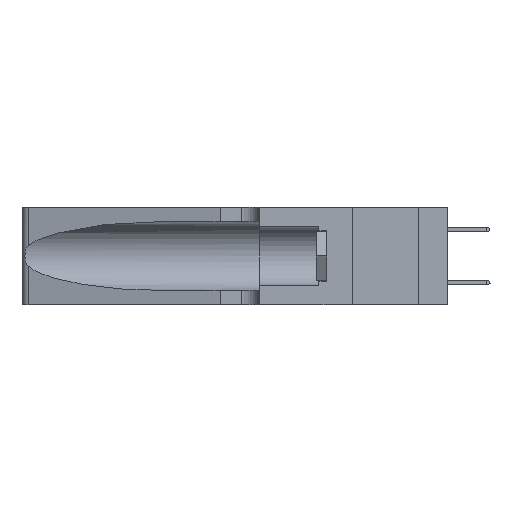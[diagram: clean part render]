
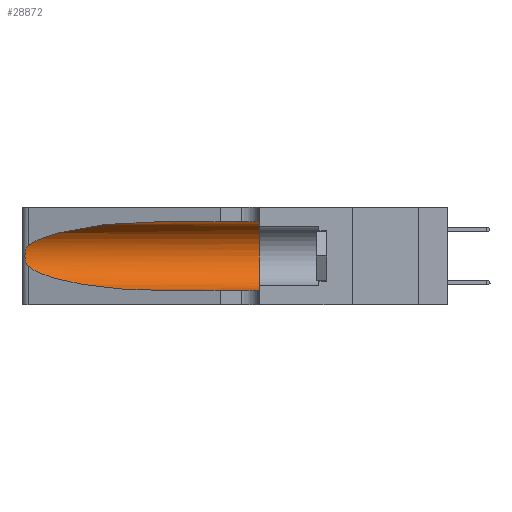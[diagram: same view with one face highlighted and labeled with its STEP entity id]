
A CAD part, left-side view. The second image highlights one B-rep face of the part: STEP entity #28872.
In plain terms, the highlighted cylindrical face has radius 3.308 mm (diameter 6.617 mm), a partial arc.
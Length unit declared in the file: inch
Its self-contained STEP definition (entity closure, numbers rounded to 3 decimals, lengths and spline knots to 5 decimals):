
#1121 = EDGE_CURVE ( 'NONE', #14903, #35474, #17194, .T. ) ;
#1436 = DIRECTION ( 'NONE',  ( 0., -1., 0. ) ) ;
#2239 =( BOUNDED_CURVE ( )  B_SPLINE_CURVE ( 3, ( #35504, #18573, #24895, #11914 ),
 .UNSPECIFIED., .F., .F. ) 
 B_SPLINE_CURVE_WITH_KNOTS ( ( 4, 4 ),
 ( 1.5708, 2.84003 ),
 .UNSPECIFIED. ) 
 CURVE ( )  GEOMETRIC_REPRESENTATION_ITEM ( )  RATIONAL_B_SPLINE_CURVE ( ( 1., 0.87, 0.87, 1. ) ) 
 REPRESENTATION_ITEM ( '' )  );
#2908 = CARTESIAN_POINT ( 'NONE',  ( 0.25487, 1.22718, 0.14631 ) ) ;
#4301 = CARTESIAN_POINT ( 'NONE',  ( 0.25789, 1.23486, 0.15765 ) ) ;
#4594 = CARTESIAN_POINT ( 'NONE',  ( 0.26075, 1.23896, 0.178 ) ) ;
#4607 = CARTESIAN_POINT ( 'NONE',  ( 0.1305, 0.72297, 0.05475 ) ) ;
#5167 = VERTEX_POINT ( 'NONE', #35663 ) ;
#6373 = EDGE_CURVE ( 'NONE', #39963, #35474, #22279, .T. ) ;
#7289 = EDGE_CURVE ( 'NONE', #42876, #39963, #41157, .T. ) ;
#7400 = EDGE_CURVE ( 'NONE', #5167, #22324, #35606, .T. ) ;
#7679 = CARTESIAN_POINT ( 'NONE',  ( 0.25555, 1.22993, 0.14849 ) ) ;
#8824 = ORIENTED_EDGE ( 'NONE', *, *, #1121, .T. ) ;
#9812 = AXIS2_PLACEMENT_3D ( 'NONE', #29751, #33416, #30193 ) ;
#10909 = CARTESIAN_POINT ( 'NONE',  ( 0.26017, 1.23833, 0.17102 ) ) ;
#11914 = CARTESIAN_POINT ( 'NONE',  ( 0.25487, 1.22718, 0.22369 ) ) ;
#13671 = EDGE_LOOP ( 'NONE', ( #27411, #39486, #29930, #8824, #27337, #23279 ) ) ;
#14017 = CARTESIAN_POINT ( 'NONE',  ( 0.25787, 1.23484, 0.2124 ) ) ;
#14903 = VERTEX_POINT ( 'NONE', #4607 ) ;
#15206 =( BOUNDED_CURVE ( )  B_SPLINE_CURVE ( 3, ( #22423, #25263, #18950, #25704 ),
 .UNSPECIFIED., .F., .F. ) 
 B_SPLINE_CURVE_WITH_KNOTS ( ( 4, 4 ),
 ( 3.44316, 4.71239 ),
 .UNSPECIFIED. ) 
 CURVE ( )  GEOMETRIC_REPRESENTATION_ITEM ( )  RATIONAL_B_SPLINE_CURVE ( ( 1., 0.87, 0.87, 1. ) ) 
 REPRESENTATION_ITEM ( '' )  );
#15389 = AXIS2_PLACEMENT_3D ( 'NONE', #18249, #1436, #25156 ) ;
#15490 = CARTESIAN_POINT ( 'NONE',  ( 0.1305, 1.61858, 0.05475 ) ) ;
#17113 = CARTESIAN_POINT ( 'NONE',  ( 0.25639, 1.23184, 0.21858 ) ) ;
#17194 = LINE ( 'NONE', #15490, #34217 ) ;
#17401 = CARTESIAN_POINT ( 'NONE',  ( 0.25854, 1.2359, 0.20912 ) ) ;
#17864 = VECTOR ( 'NONE', #36805, 39.37008 ) ;
#18249 = CARTESIAN_POINT ( 'NONE',  ( 0.1305, 1.61858, 0.185 ) ) ;
#18559 = CYLINDRICAL_SURFACE ( 'NONE', #15389, 0.13025 ) ;
#18573 = CARTESIAN_POINT ( 'NONE',  ( 0.18966, 0.96281, 0.31525 ) ) ;
#18950 = CARTESIAN_POINT ( 'NONE',  ( 0.18966, 0.96281, 0.05475 ) ) ;
#20403 = CARTESIAN_POINT ( 'NONE',  ( 0.1305, 0.35, 0.31525 ) ) ;
#20869 = CARTESIAN_POINT ( 'NONE',  ( 0.25555, 1.22994, 0.2215 ) ) ;
#22206 = EDGE_CURVE ( 'NONE', #42876, #5167, #2239, .T. ) ;
#22279 = CIRCLE ( 'NONE', #9812, 0.13025 ) ;
#22324 = VERTEX_POINT ( 'NONE', #2908 ) ;
#22423 = CARTESIAN_POINT ( 'NONE',  ( 0.25487, 1.22718, 0.14631 ) ) ;
#23279 = ORIENTED_EDGE ( 'NONE', *, *, #7289, .F. ) ;
#24479 = CARTESIAN_POINT ( 'NONE',  ( 0.26018, 1.23835, 0.19895 ) ) ;
#24771 = CARTESIAN_POINT ( 'NONE',  ( 0.25639, 1.23186, 0.15144 ) ) ;
#24895 = CARTESIAN_POINT ( 'NONE',  ( 0.2373, 1.15595, 0.28018 ) ) ;
#25156 = DIRECTION ( 'NONE',  ( 0., 0., -1. ) ) ;
#25263 = CARTESIAN_POINT ( 'NONE',  ( 0.2373, 1.15595, 0.08982 ) ) ;
#25704 = CARTESIAN_POINT ( 'NONE',  ( 0.1305, 0.72297, 0.05475 ) ) ;
#27337 = ORIENTED_EDGE ( 'NONE', *, *, #6373, .F. ) ;
#27411 = ORIENTED_EDGE ( 'NONE', *, *, #22206, .T. ) ;
#28740 = FACE_OUTER_BOUND ( 'NONE', #13671, .T. ) ;
#28872 = ADVANCED_FACE ( 'NONE', ( #28740 ), #18559, .F. ) ;
#29751 = CARTESIAN_POINT ( 'NONE',  ( 0.1305, 0.35, 0.185 ) ) ;
#29930 = ORIENTED_EDGE ( 'NONE', *, *, #33327, .T. ) ;
#29977 = CARTESIAN_POINT ( 'NONE',  ( 0.1305, 0.35, 0.05475 ) ) ;
#30193 = DIRECTION ( 'NONE',  ( 0., 0., 1. ) ) ;
#31260 = CARTESIAN_POINT ( 'NONE',  ( 0.26075, 1.23896, 0.19203 ) ) ;
#31564 = CARTESIAN_POINT ( 'NONE',  ( 0.25487, 1.22718, 0.14631 ) ) ;
#32302 = DIRECTION ( 'NONE',  ( 0., -1., 0. ) ) ;
#33327 = EDGE_CURVE ( 'NONE', #22324, #14903, #15206, .T. ) ;
#33416 = DIRECTION ( 'NONE',  ( 0., 1., 0. ) ) ;
#34217 = VECTOR ( 'NONE', #32302, 39.37008 ) ;
#35474 = VERTEX_POINT ( 'NONE', #29977 ) ;
#35504 = CARTESIAN_POINT ( 'NONE',  ( 0.1305, 0.72297, 0.31525 ) ) ;
#35606 = B_SPLINE_CURVE_WITH_KNOTS ( 'NONE', 3,
 ( #43207, #20869, #17113, #14017, #17401, #24479, #31260, #4594, #10909, #41401, #4301, #24771, #7679, #31564 ),
 .UNSPECIFIED., .F., .F.,
 ( 4, 2, 2, 2, 2, 2, 4 ),
 ( 0., 0.00027, 0.00053, 0.00107, 0.0016, 0.00187, 0.00214 ),
 .UNSPECIFIED. ) ;
#35663 = CARTESIAN_POINT ( 'NONE',  ( 0.25487, 1.22718, 0.22369 ) ) ;
#36296 = CARTESIAN_POINT ( 'NONE',  ( 0.1305, 0.72297, 0.31525 ) ) ;
#36805 = DIRECTION ( 'NONE',  ( 0., -1., 0. ) ) ;
#39486 = ORIENTED_EDGE ( 'NONE', *, *, #7400, .T. ) ;
#39963 = VERTEX_POINT ( 'NONE', #20403 ) ;
#41157 = LINE ( 'NONE', #42214, #17864 ) ;
#41401 = CARTESIAN_POINT ( 'NONE',  ( 0.25856, 1.23593, 0.16098 ) ) ;
#42214 = CARTESIAN_POINT ( 'NONE',  ( 0.1305, 1.61858, 0.31525 ) ) ;
#42876 = VERTEX_POINT ( 'NONE', #36296 ) ;
#43207 = CARTESIAN_POINT ( 'NONE',  ( 0.25487, 1.22718, 0.22369 ) ) ;
